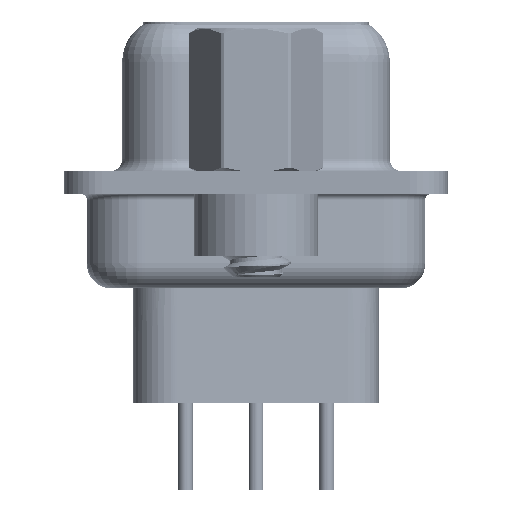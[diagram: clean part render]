
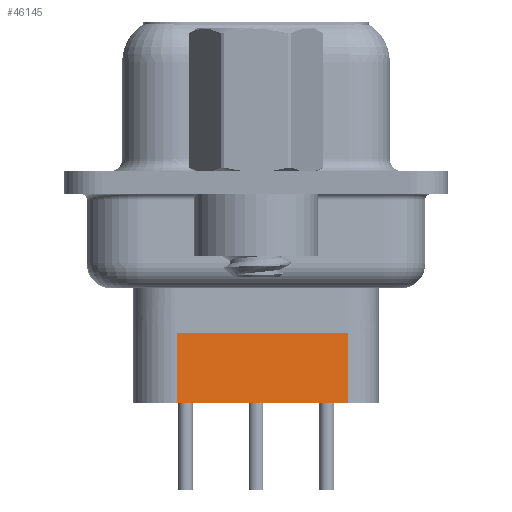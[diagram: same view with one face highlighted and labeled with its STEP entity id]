
A CAD part, left-side view. The second image highlights one B-rep face of the part: STEP entity #46145.
In plain terms, the highlighted planar face has unit normal (-0.985, -0.174, 0).
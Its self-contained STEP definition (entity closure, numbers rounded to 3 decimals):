
#1925 = DIRECTION ( 'NONE',  ( 0.174, -0.985, 0. ) ) ;
#2241 = VECTOR ( 'NONE', #39886, 1000. ) ;
#3763 = ORIENTED_EDGE ( 'NONE', *, *, #4204, .T. ) ;
#3790 = AXIS2_PLACEMENT_3D ( 'NONE', #8870, #16843, #1925 ) ;
#4204 = EDGE_CURVE ( 'NONE', #47731, #6369, #16501, .T. ) ;
#5292 = CARTESIAN_POINT ( 'NONE',  ( 5.781, -3.685, -6.05 ) ) ;
#6369 = VERTEX_POINT ( 'NONE', #26624 ) ;
#7163 = LINE ( 'NONE', #33646, #25754 ) ;
#7773 = CARTESIAN_POINT ( 'NONE',  ( 4.574, 3.165, -3.1 ) ) ;
#8641 = CARTESIAN_POINT ( 'NONE',  ( 4.574, 3.165, -6.05 ) ) ;
#8870 = CARTESIAN_POINT ( 'NONE',  ( 4.574, 3.165, -3.1 ) ) ;
#10340 = LINE ( 'NONE', #8641, #20724 ) ;
#11217 = EDGE_CURVE ( 'NONE', #14027, #46737, #7163, .T. ) ;
#12749 = DIRECTION ( 'NONE',  ( -0.174, 0.985, 0. ) ) ;
#14027 = VERTEX_POINT ( 'NONE', #5292 ) ;
#15499 = ORIENTED_EDGE ( 'NONE', *, *, #33543, .T. ) ;
#16501 = LINE ( 'NONE', #7773, #2241 ) ;
#16843 = DIRECTION ( 'NONE',  ( -0.985, -0.174, 0. ) ) ;
#17390 = CARTESIAN_POINT ( 'NONE',  ( 4.574, 3.165, -8.85 ) ) ;
#20253 = ORIENTED_EDGE ( 'NONE', *, *, #23727, .F. ) ;
#20724 = VECTOR ( 'NONE', #12749, 1000. ) ;
#21753 = DIRECTION ( 'NONE',  ( -0.174, 0.985, 0. ) ) ;
#23727 = EDGE_CURVE ( 'NONE', #46737, #6369, #25339, .T. ) ;
#23796 = EDGE_LOOP ( 'NONE', ( #43253, #15499, #3763, #20253 ) ) ;
#25339 = LINE ( 'NONE', #17390, #39043 ) ;
#25519 = CARTESIAN_POINT ( 'NONE',  ( 5.781, -3.685, -8.85 ) ) ;
#25754 = VECTOR ( 'NONE', #30040, 1000. ) ;
#26624 = CARTESIAN_POINT ( 'NONE',  ( 4.574, 3.165, -8.85 ) ) ;
#30040 = DIRECTION ( 'NONE',  ( 0., 0., -1. ) ) ;
#31519 = FACE_OUTER_BOUND ( 'NONE', #23796, .T. ) ;
#33543 = EDGE_CURVE ( 'NONE', #14027, #47731, #10340, .T. ) ;
#33646 = CARTESIAN_POINT ( 'NONE',  ( 5.781, -3.685, -3.1 ) ) ;
#39043 = VECTOR ( 'NONE', #21753, 1000. ) ;
#39886 = DIRECTION ( 'NONE',  ( 0., 0., -1. ) ) ;
#43253 = ORIENTED_EDGE ( 'NONE', *, *, #11217, .F. ) ;
#46145 = ADVANCED_FACE ( 'NONE', ( #31519 ), #47157, .T. ) ;
#46175 = CARTESIAN_POINT ( 'NONE',  ( 4.574, 3.165, -6.05 ) ) ;
#46737 = VERTEX_POINT ( 'NONE', #25519 ) ;
#47157 = PLANE ( 'NONE',  #3790 ) ;
#47731 = VERTEX_POINT ( 'NONE', #46175 ) ;
